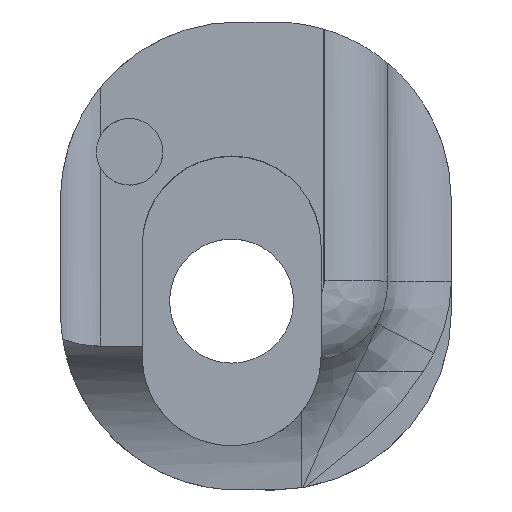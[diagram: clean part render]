
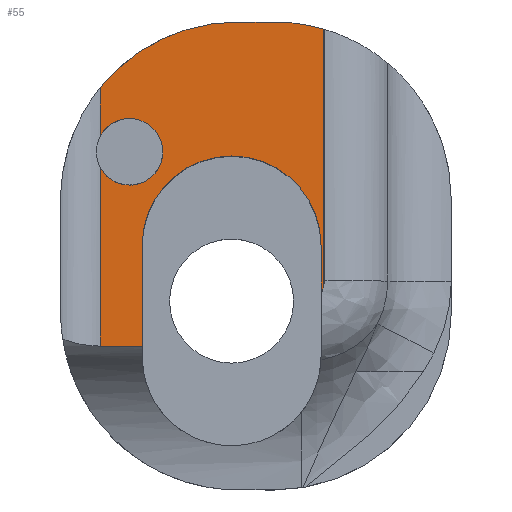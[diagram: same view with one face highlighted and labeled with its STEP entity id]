
A CAD part, top view. The second image highlights one B-rep face of the part: STEP entity #55.
In plain terms, the highlighted planar face has unit normal (0, 0, 1).
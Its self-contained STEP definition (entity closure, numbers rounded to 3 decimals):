
#19 = CARTESIAN_POINT ( 'NONE',  ( 75.363, 12.557, 49.76 ) ) ;
#24 = ORIENTED_EDGE ( 'NONE', *, *, #1293, .F. ) ;
#32 = VECTOR ( 'NONE', #522, 1000. ) ;
#38 = DIRECTION ( 'NONE',  ( 1., 0., 0. ) ) ;
#40 = CARTESIAN_POINT ( 'NONE',  ( 57.11, 17.102, 49.76 ) ) ;
#47 = DIRECTION ( 'NONE',  ( 0., -1., 0. ) ) ;
#55 = ADVANCED_FACE ( 'NONE', ( #710 ), #807, .F. ) ;
#116 = CARTESIAN_POINT ( 'NONE',  ( 61.148, 0.312, 49.76 ) ) ;
#124 = VERTEX_POINT ( 'NONE', #963 ) ;
#137 = ORIENTED_EDGE ( 'NONE', *, *, #402, .F. ) ;
#145 = DIRECTION ( 'NONE',  ( 1., 0., 0. ) ) ;
#155 = VERTEX_POINT ( 'NONE', #986 ) ;
#167 = CIRCLE ( 'NONE', #1123, 1.5 ) ;
#173 = DIRECTION ( 'NONE',  ( 1., 0., 0. ) ) ;
#201 = CARTESIAN_POINT ( 'NONE',  ( 51.172, 24.223, 49.76 ) ) ;
#231 = DIRECTION ( 'NONE',  ( 0., 0., 1. ) ) ;
#234 = AXIS2_PLACEMENT_3D ( 'NONE', #1014, #231, #1138 ) ;
#250 = CIRCLE ( 'NONE', #234, 8. ) ;
#251 = EDGE_CURVE ( 'NONE', #155, #316, #689, .T. ) ;
#257 = VECTOR ( 'NONE', #1451, 1000. ) ;
#260 = CARTESIAN_POINT ( 'NONE',  ( 53.071, 12.557, 49.76 ) ) ;
#294 = ORIENTED_EDGE ( 'NONE', *, *, #251, .T. ) ;
#298 = VECTOR ( 'NONE', #145, 1000. ) ;
#300 = CARTESIAN_POINT ( 'NONE',  ( 52.502, 21.324, 49.76 ) ) ;
#309 = EDGE_CURVE ( 'NONE', #782, #316, #331, .T. ) ;
#315 = CARTESIAN_POINT ( 'NONE',  ( 51.172, 24.67, 49.76 ) ) ;
#316 = VERTEX_POINT ( 'NONE', #1423 ) ;
#331 = LINE ( 'NONE', #1219, #1324 ) ;
#357 = VERTEX_POINT ( 'NONE', #977 ) ;
#370 = DIRECTION ( 'NONE',  ( 0., 1., 0. ) ) ;
#402 = EDGE_CURVE ( 'NONE', #124, #648, #612, .T. ) ;
#419 = EDGE_CURVE ( 'NONE', #1064, #782, #1584, .T. ) ;
#422 = ORIENTED_EDGE ( 'NONE', *, *, #419, .F. ) ;
#446 = EDGE_CURVE ( 'NONE', #751, #155, #167, .T. ) ;
#454 = LINE ( 'NONE', #116, #1101 ) ;
#457 = DIRECTION ( 'NONE',  ( 0., 0., -1. ) ) ;
#489 = VERTEX_POINT ( 'NONE', #1591 ) ;
#490 = CARTESIAN_POINT ( 'NONE',  ( 57.391, 27.191, 49.76 ) ) ;
#510 = CARTESIAN_POINT ( 'NONE',  ( 59.033, 19.191, 49.76 ) ) ;
#513 = CARTESIAN_POINT ( 'NONE',  ( 51.172, 22.018, 49.76 ) ) ;
#522 = DIRECTION ( 'NONE',  ( 0., -1., 0. ) ) ;
#539 = CARTESIAN_POINT ( 'NONE',  ( 61.269, 15.279, 49.76 ) ) ;
#544 = DIRECTION ( 'NONE',  ( 0., 1., 0. ) ) ;
#550 = DIRECTION ( 'NONE',  ( 0., 0., -1. ) ) ;
#582 = CIRCLE ( 'NONE', #704, 8. ) ;
#612 = B_SPLINE_CURVE_WITH_KNOTS ( 'NONE', 3,
 ( #1189, #539, #1447, #684, #1577, #814 ),
 .UNSPECIFIED., .F., .F.,
 ( 4, 2, 4 ),
 ( 0., 0., 0.001 ),
 .UNSPECIFIED. ) ;
#646 = DIRECTION ( 'NONE',  ( 1., 0., 0. ) ) ;
#648 = VERTEX_POINT ( 'NONE', #1009 ) ;
#657 = LINE ( 'NONE', #799, #298 ) ;
#684 = CARTESIAN_POINT ( 'NONE',  ( 61.228, 15.091, 49.76 ) ) ;
#685 = DIRECTION ( 'NONE',  ( 1., 0., 0. ) ) ;
#689 = CIRCLE ( 'NONE', #1642, 1.5 ) ;
#692 = ORIENTED_EDGE ( 'NONE', *, *, #1605, .T. ) ;
#704 = AXIS2_PLACEMENT_3D ( 'NONE', #510, #1418, #646 ) ;
#710 = FACE_OUTER_BOUND ( 'NONE', #1588, .T. ) ;
#718 = ORIENTED_EDGE ( 'NONE', *, *, #446, .T. ) ;
#725 = EDGE_CURVE ( 'NONE', #357, #845, #582, .T. ) ;
#751 = VERTEX_POINT ( 'NONE', #513 ) ;
#767 = LINE ( 'NONE', #315, #1051 ) ;
#782 = VERTEX_POINT ( 'NONE', #1435 ) ;
#799 = CARTESIAN_POINT ( 'NONE',  ( 135.443, 27.191, 49.76 ) ) ;
#807 = PLANE ( 'NONE',  #1419 ) ;
#814 = CARTESIAN_POINT ( 'NONE',  ( 61.148, 14.899, 49.76 ) ) ;
#835 = VECTOR ( 'NONE', #47, 1000. ) ;
#845 = VERTEX_POINT ( 'NONE', #1185 ) ;
#959 = DIRECTION ( 'NONE',  ( 0., 0., 1. ) ) ;
#963 = CARTESIAN_POINT ( 'NONE',  ( 61.275, 15.324, 49.76 ) ) ;
#966 = EDGE_CURVE ( 'NONE', #648, #489, #454, .T. ) ;
#977 = CARTESIAN_POINT ( 'NONE',  ( 61.274, 26.87, 49.76 ) ) ;
#986 = CARTESIAN_POINT ( 'NONE',  ( 54.002, 21.324, 49.76 ) ) ;
#988 = CARTESIAN_POINT ( 'NONE',  ( 53.071, 17.102, 49.76 ) ) ;
#1009 = CARTESIAN_POINT ( 'NONE',  ( 61.148, 14.899, 49.76 ) ) ;
#1014 = CARTESIAN_POINT ( 'NONE',  ( 57.391, 19.191, 49.76 ) ) ;
#1040 = ORIENTED_EDGE ( 'NONE', *, *, #1090, .F. ) ;
#1051 = VECTOR ( 'NONE', #1359, 1000. ) ;
#1064 = VERTEX_POINT ( 'NONE', #260 ) ;
#1090 = EDGE_CURVE ( 'NONE', #357, #124, #1112, .T. ) ;
#1101 = VECTOR ( 'NONE', #370, 1000. ) ;
#1112 = LINE ( 'NONE', #1557, #32 ) ;
#1114 = ORIENTED_EDGE ( 'NONE', *, *, #309, .F. ) ;
#1123 = AXIS2_PLACEMENT_3D ( 'NONE', #1328, #550, #1454 ) ;
#1138 = DIRECTION ( 'NONE',  ( 1., 0., 0. ) ) ;
#1159 = AXIS2_PLACEMENT_3D ( 'NONE', #40, #959, #173 ) ;
#1162 = EDGE_CURVE ( 'NONE', #1612, #845, #657, .T. ) ;
#1168 = CARTESIAN_POINT ( 'NONE',  ( 135.443, 0.312, 49.76 ) ) ;
#1173 = LINE ( 'NONE', #1344, #835 ) ;
#1185 = CARTESIAN_POINT ( 'NONE',  ( 59.033, 27.191, 49.76 ) ) ;
#1189 = CARTESIAN_POINT ( 'NONE',  ( 61.275, 15.324, 49.76 ) ) ;
#1219 = CARTESIAN_POINT ( 'NONE',  ( 51.172, 24.67, 49.76 ) ) ;
#1267 = EDGE_CURVE ( 'NONE', #489, #1561, #1593, .T. ) ;
#1269 = ORIENTED_EDGE ( 'NONE', *, *, #1267, .F. ) ;
#1293 = EDGE_CURVE ( 'NONE', #1561, #1064, #1173, .T. ) ;
#1324 = VECTOR ( 'NONE', #544, 1000. ) ;
#1328 = CARTESIAN_POINT ( 'NONE',  ( 52.502, 21.324, 49.76 ) ) ;
#1329 = DIRECTION ( 'NONE',  ( 0., 0., -1. ) ) ;
#1344 = CARTESIAN_POINT ( 'NONE',  ( 53.071, 0.312, 49.76 ) ) ;
#1359 = DIRECTION ( 'NONE',  ( 0., 1., 0. ) ) ;
#1418 = DIRECTION ( 'NONE',  ( 0., 0., 1. ) ) ;
#1419 = AXIS2_PLACEMENT_3D ( 'NONE', #1168, #1329, #685 ) ;
#1423 = CARTESIAN_POINT ( 'NONE',  ( 51.172, 20.631, 49.76 ) ) ;
#1424 = ORIENTED_EDGE ( 'NONE', *, *, #725, .T. ) ;
#1431 = ORIENTED_EDGE ( 'NONE', *, *, #966, .F. ) ;
#1435 = CARTESIAN_POINT ( 'NONE',  ( 51.172, 12.557, 49.76 ) ) ;
#1438 = EDGE_CURVE ( 'NONE', #751, #1522, #767, .T. ) ;
#1447 = CARTESIAN_POINT ( 'NONE',  ( 61.261, 15.235, 49.76 ) ) ;
#1451 = DIRECTION ( 'NONE',  ( -1., 0., 0. ) ) ;
#1454 = DIRECTION ( 'NONE',  ( 1., 0., 0. ) ) ;
#1517 = ORIENTED_EDGE ( 'NONE', *, *, #1162, .F. ) ;
#1522 = VERTEX_POINT ( 'NONE', #201 ) ;
#1557 = CARTESIAN_POINT ( 'NONE',  ( 61.274, 15.497, 49.76 ) ) ;
#1561 = VERTEX_POINT ( 'NONE', #988 ) ;
#1577 = CARTESIAN_POINT ( 'NONE',  ( 61.194, 14.992, 49.76 ) ) ;
#1584 = LINE ( 'NONE', #19, #257 ) ;
#1586 = ORIENTED_EDGE ( 'NONE', *, *, #1438, .F. ) ;
#1588 = EDGE_LOOP ( 'NONE', ( #1040, #1424, #1517, #692, #1586, #718, #294, #1114, #422, #24, #1269, #1431, #137 ) ) ;
#1591 = CARTESIAN_POINT ( 'NONE',  ( 61.148, 17.102, 49.76 ) ) ;
#1593 = CIRCLE ( 'NONE', #1159, 4.039 ) ;
#1605 = EDGE_CURVE ( 'NONE', #1612, #1522, #250, .T. ) ;
#1612 = VERTEX_POINT ( 'NONE', #490 ) ;
#1642 = AXIS2_PLACEMENT_3D ( 'NONE', #300, #457, #38 ) ;
